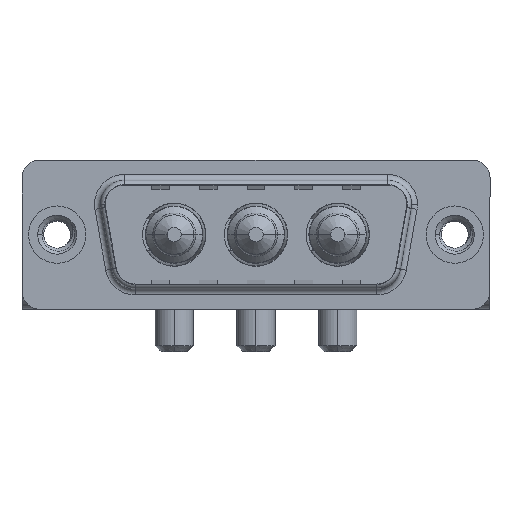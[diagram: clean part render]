
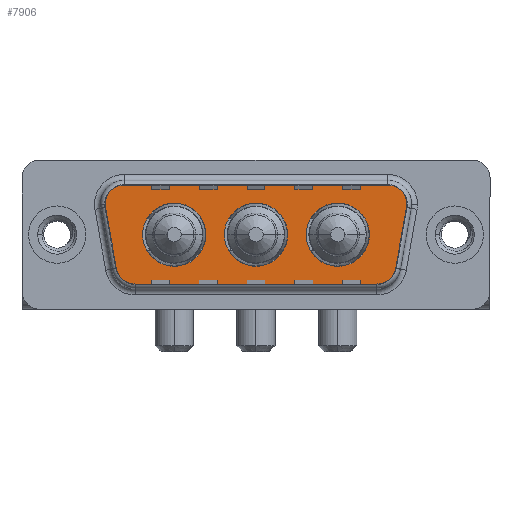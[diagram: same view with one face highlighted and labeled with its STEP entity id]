
A CAD part, top view. The second image highlights one B-rep face of the part: STEP entity #7906.
In plain terms, the highlighted planar face has unit normal (0, 0, 1).
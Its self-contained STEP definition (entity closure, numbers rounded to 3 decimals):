
#20 = FACE_BOUND ( 'NONE', #12363, .T. ) ;
#97 = AXIS2_PLACEMENT_3D ( 'NONE', #2376, #7723, #11974 ) ;
#133 = VERTEX_POINT ( 'NONE', #9998 ) ;
#184 = DIRECTION ( 'NONE',  ( 0., 0., 1. ) ) ;
#216 = EDGE_CURVE ( 'NONE', #2985, #7086, #13813, .T. ) ;
#265 = VERTEX_POINT ( 'NONE', #4590 ) ;
#307 = LINE ( 'NONE', #12158, #1023 ) ;
#332 = EDGE_CURVE ( 'NONE', #133, #2985, #649, .T. ) ;
#375 = ORIENTED_EDGE ( 'NONE', *, *, #6806, .F. ) ;
#484 = AXIS2_PLACEMENT_3D ( 'NONE', #5494, #11802, #9776 ) ;
#520 = DIRECTION ( 'NONE',  ( 0., 0., 1. ) ) ;
#563 = VERTEX_POINT ( 'NONE', #11730 ) ;
#649 = LINE ( 'NONE', #3743, #9821 ) ;
#744 = AXIS2_PLACEMENT_3D ( 'NONE', #12357, #10211, #2761 ) ;
#842 = CARTESIAN_POINT ( 'NONE',  ( 6.434, -4.9, 0. ) ) ;
#964 = ORIENTED_EDGE ( 'NONE', *, *, #1806, .T. ) ;
#1023 = VECTOR ( 'NONE', #6912, 1000. ) ;
#1065 = DIRECTION ( 'NONE',  ( 0.174, 0.985, 0. ) ) ;
#1154 = AXIS2_PLACEMENT_3D ( 'NONE', #11385, #10412, #1854 ) ;
#1184 = EDGE_LOOP ( 'NONE', ( #7975, #6429 ) ) ;
#1324 = DIRECTION ( 'NONE',  ( 0., 0., 1. ) ) ;
#1545 = ORIENTED_EDGE ( 'NONE', *, *, #5651, .T. ) ;
#1806 = EDGE_CURVE ( 'NONE', #7086, #6479, #8500, .T. ) ;
#1854 = DIRECTION ( 'NONE',  ( 1., 0., 0. ) ) ;
#1895 = ORIENTED_EDGE ( 'NONE', *, *, #10657, .T. ) ;
#1995 = EDGE_CURVE ( 'NONE', #265, #11484, #3808, .T. ) ;
#2123 = VECTOR ( 'NONE', #1065, 1000. ) ;
#2376 = CARTESIAN_POINT ( 'NONE',  ( 9.8, 0., 0. ) ) ;
#2452 = CARTESIAN_POINT ( 'NONE',  ( 16.65, 0., 0. ) ) ;
#2621 = DIRECTION ( 'NONE',  ( 1., 0., 0. ) ) ;
#2761 = DIRECTION ( 'NONE',  ( 1., 0., 0. ) ) ;
#2766 = ORIENTED_EDGE ( 'NONE', *, *, #11794, .T. ) ;
#2951 = AXIS2_PLACEMENT_3D ( 'NONE', #2452, #10926, #9972 ) ;
#2985 = VERTEX_POINT ( 'NONE', #5233 ) ;
#2995 = CARTESIAN_POINT ( 'NONE',  ( 27.889, 4.9, 0. ) ) ;
#3030 = CARTESIAN_POINT ( 'NONE',  ( 12.45, 0., 0. ) ) ;
#3301 = EDGE_CURVE ( 'NONE', #11484, #265, #8999, .T. ) ;
#3305 = LINE ( 'NONE', #5204, #2123 ) ;
#3315 = PLANE ( 'NONE',  #10651 ) ;
#3533 = CIRCLE ( 'NONE', #13581, 2.65 ) ;
#3674 = DIRECTION ( 'NONE',  ( 0., 0., 1. ) ) ;
#3743 = CARTESIAN_POINT ( 'NONE',  ( 3.441, 2.553, 0. ) ) ;
#3808 = CIRCLE ( 'NONE', #5596, 2.65 ) ;
#4296 = DIRECTION ( 'NONE',  ( 1., 0., 0. ) ) ;
#4534 = EDGE_CURVE ( 'NONE', #8378, #5338, #7923, .T. ) ;
#4590 = CARTESIAN_POINT ( 'NONE',  ( 14., 0., 0. ) ) ;
#4803 = DIRECTION ( 'NONE',  ( -1., 0., 0. ) ) ;
#5186 = VERTEX_POINT ( 'NONE', #9077 ) ;
#5204 = CARTESIAN_POINT ( 'NONE',  ( 29.859, 2.553, 0. ) ) ;
#5233 = CARTESIAN_POINT ( 'NONE',  ( 4.464, -3.247, 0. ) ) ;
#5338 = VERTEX_POINT ( 'NONE', #11063 ) ;
#5374 = VECTOR ( 'NONE', #11715, 1000. ) ;
#5378 = CARTESIAN_POINT ( 'NONE',  ( 29.859, 2.553, 0. ) ) ;
#5410 = CIRCLE ( 'NONE', #1154, 2.65 ) ;
#5494 = CARTESIAN_POINT ( 'NONE',  ( 27.889, 2.9, 0. ) ) ;
#5596 = AXIS2_PLACEMENT_3D ( 'NONE', #10921, #1324, #5603 ) ;
#5603 = DIRECTION ( 'NONE',  ( 1., 0., 0. ) ) ;
#5650 = ORIENTED_EDGE ( 'NONE', *, *, #3301, .F. ) ;
#5651 = EDGE_CURVE ( 'NONE', #6479, #7523, #11733, .T. ) ;
#6097 = CARTESIAN_POINT ( 'NONE',  ( 26.15, 0., 0. ) ) ;
#6429 = ORIENTED_EDGE ( 'NONE', *, *, #10442, .F. ) ;
#6433 = ORIENTED_EDGE ( 'NONE', *, *, #216, .T. ) ;
#6479 = VERTEX_POINT ( 'NONE', #7125 ) ;
#6773 = CARTESIAN_POINT ( 'NONE',  ( 27.889, 2.9, 0. ) ) ;
#6806 = EDGE_CURVE ( 'NONE', #12293, #5186, #3533, .T. ) ;
#6912 = DIRECTION ( 'NONE',  ( -1., 0., 0. ) ) ;
#7086 = VERTEX_POINT ( 'NONE', #842 ) ;
#7125 = CARTESIAN_POINT ( 'NONE',  ( 26.866, -4.9, 0. ) ) ;
#7402 = CARTESIAN_POINT ( 'NONE',  ( 26.866, -2.9, 0. ) ) ;
#7455 = CARTESIAN_POINT ( 'NONE',  ( 6.434, -4.9, 0. ) ) ;
#7523 = VERTEX_POINT ( 'NONE', #8730 ) ;
#7546 = FACE_OUTER_BOUND ( 'NONE', #9368, .T. ) ;
#7555 = EDGE_LOOP ( 'NONE', ( #5650, #8380 ) ) ;
#7596 = EDGE_CURVE ( 'NONE', #8578, #563, #10207, .T. ) ;
#7633 = EDGE_CURVE ( 'NONE', #10021, #9996, #307, .T. ) ;
#7655 = ORIENTED_EDGE ( 'NONE', *, *, #332, .T. ) ;
#7723 = DIRECTION ( 'NONE',  ( 0., 0., 1. ) ) ;
#7820 = AXIS2_PLACEMENT_3D ( 'NONE', #13258, #3674, #12153 ) ;
#7906 = ADVANCED_FACE ( 'NONE', ( #10670, #8515, #20, #7546 ), #3315, .T. ) ;
#7909 = DIRECTION ( 'NONE',  ( 0., 0., 1. ) ) ;
#7918 = ORIENTED_EDGE ( 'NONE', *, *, #13586, .T. ) ;
#7923 = CIRCLE ( 'NONE', #11708, 2.65 ) ;
#7975 = ORIENTED_EDGE ( 'NONE', *, *, #4534, .F. ) ;
#8378 = VERTEX_POINT ( 'NONE', #6097 ) ;
#8380 = ORIENTED_EDGE ( 'NONE', *, *, #1995, .F. ) ;
#8500 = LINE ( 'NONE', #7455, #5374 ) ;
#8515 = FACE_BOUND ( 'NONE', #1184, .T. ) ;
#8578 = VERTEX_POINT ( 'NONE', #5378 ) ;
#8730 = CARTESIAN_POINT ( 'NONE',  ( 28.836, -3.247, 0. ) ) ;
#8785 = CARTESIAN_POINT ( 'NONE',  ( 9.8, 0., 0. ) ) ;
#8999 = CIRCLE ( 'NONE', #2951, 2.65 ) ;
#9077 = CARTESIAN_POINT ( 'NONE',  ( 7.15, 0., 0. ) ) ;
#9175 = ORIENTED_EDGE ( 'NONE', *, *, #12895, .F. ) ;
#9368 = EDGE_LOOP ( 'NONE', ( #1545, #7918, #11565, #1895, #10699, #2766, #7655, #6433, #964 ) ) ;
#9540 = AXIS2_PLACEMENT_3D ( 'NONE', #6773, #520, #4803 ) ;
#9598 = CARTESIAN_POINT ( 'NONE',  ( 26.866, -2.9, 0. ) ) ;
#9776 = DIRECTION ( 'NONE',  ( -1., 0., 0. ) ) ;
#9821 = VECTOR ( 'NONE', #10464, 1000. ) ;
#9972 = DIRECTION ( 'NONE',  ( 1., 0., 0. ) ) ;
#9996 = VERTEX_POINT ( 'NONE', #12503 ) ;
#9998 = CARTESIAN_POINT ( 'NONE',  ( 3.441, 2.553, 0. ) ) ;
#10021 = VERTEX_POINT ( 'NONE', #2995 ) ;
#10178 = CIRCLE ( 'NONE', #97, 2.65 ) ;
#10207 = CIRCLE ( 'NONE', #9540, 2. ) ;
#10211 = DIRECTION ( 'NONE',  ( 0., 0., 1. ) ) ;
#10412 = DIRECTION ( 'NONE',  ( 0., 0., 1. ) ) ;
#10442 = EDGE_CURVE ( 'NONE', #5338, #8378, #5410, .T. ) ;
#10464 = DIRECTION ( 'NONE',  ( 0.174, -0.985, 0. ) ) ;
#10651 = AXIS2_PLACEMENT_3D ( 'NONE', #7402, #11657, #4296 ) ;
#10657 = EDGE_CURVE ( 'NONE', #563, #10021, #11684, .T. ) ;
#10670 = FACE_BOUND ( 'NONE', #7555, .T. ) ;
#10699 = ORIENTED_EDGE ( 'NONE', *, *, #7633, .T. ) ;
#10700 = DIRECTION ( 'NONE',  ( 1., 0., 0. ) ) ;
#10921 = CARTESIAN_POINT ( 'NONE',  ( 16.65, 0., 0. ) ) ;
#10926 = DIRECTION ( 'NONE',  ( 0., 0., 1. ) ) ;
#11063 = CARTESIAN_POINT ( 'NONE',  ( 20.85, 0., 0. ) ) ;
#11385 = CARTESIAN_POINT ( 'NONE',  ( 23.5, 0., 0. ) ) ;
#11484 = VERTEX_POINT ( 'NONE', #12648 ) ;
#11565 = ORIENTED_EDGE ( 'NONE', *, *, #7596, .T. ) ;
#11657 = DIRECTION ( 'NONE',  ( 0., 0., 1. ) ) ;
#11684 = CIRCLE ( 'NONE', #484, 2. ) ;
#11708 = AXIS2_PLACEMENT_3D ( 'NONE', #12223, #7909, #2621 ) ;
#11715 = DIRECTION ( 'NONE',  ( 1., 0., 0. ) ) ;
#11730 = CARTESIAN_POINT ( 'NONE',  ( 29.889, 2.9, 0. ) ) ;
#11733 = CIRCLE ( 'NONE', #12385, 2. ) ;
#11794 = EDGE_CURVE ( 'NONE', #9996, #133, #12817, .T. ) ;
#11802 = DIRECTION ( 'NONE',  ( 0., 0., 1. ) ) ;
#11974 = DIRECTION ( 'NONE',  ( 1., 0., 0. ) ) ;
#12153 = DIRECTION ( 'NONE',  ( -1., 0., 0. ) ) ;
#12158 = CARTESIAN_POINT ( 'NONE',  ( 5.411, 4.9, 0. ) ) ;
#12208 = DIRECTION ( 'NONE',  ( 1., 0., 0. ) ) ;
#12223 = CARTESIAN_POINT ( 'NONE',  ( 23.5, 0., 0. ) ) ;
#12293 = VERTEX_POINT ( 'NONE', #3030 ) ;
#12357 = CARTESIAN_POINT ( 'NONE',  ( 5.411, 2.9, 0. ) ) ;
#12363 = EDGE_LOOP ( 'NONE', ( #375, #9175 ) ) ;
#12385 = AXIS2_PLACEMENT_3D ( 'NONE', #9598, #184, #10700 ) ;
#12503 = CARTESIAN_POINT ( 'NONE',  ( 5.411, 4.9, 0. ) ) ;
#12648 = CARTESIAN_POINT ( 'NONE',  ( 19.3, 0., 0. ) ) ;
#12817 = CIRCLE ( 'NONE', #744, 2. ) ;
#12895 = EDGE_CURVE ( 'NONE', #5186, #12293, #10178, .T. ) ;
#13037 = DIRECTION ( 'NONE',  ( 0., 0., 1. ) ) ;
#13258 = CARTESIAN_POINT ( 'NONE',  ( 6.434, -2.9, 0. ) ) ;
#13581 = AXIS2_PLACEMENT_3D ( 'NONE', #8785, #13037, #12208 ) ;
#13586 = EDGE_CURVE ( 'NONE', #7523, #8578, #3305, .T. ) ;
#13813 = CIRCLE ( 'NONE', #7820, 2. ) ;
